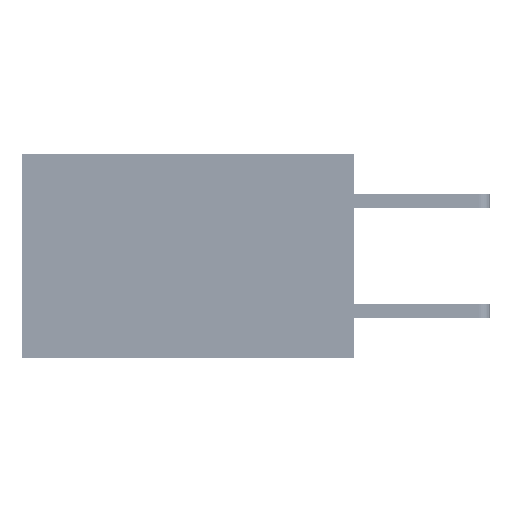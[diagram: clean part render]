
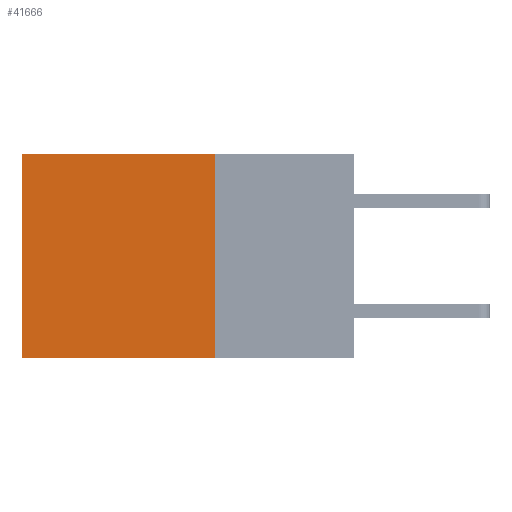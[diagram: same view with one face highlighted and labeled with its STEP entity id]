
A CAD part, left-side view. The second image highlights one B-rep face of the part: STEP entity #41666.
In plain terms, the highlighted planar face has unit normal (-1, 0, 0).
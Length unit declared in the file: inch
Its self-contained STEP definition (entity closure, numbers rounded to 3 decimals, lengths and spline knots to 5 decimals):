
#1092 = ORIENTED_EDGE ( 'NONE', *, *, #19078, .F. ) ;
#1303 = ORIENTED_EDGE ( 'NONE', *, *, #3907, .T. ) ;
#3804 = CARTESIAN_POINT ( 'NONE',  ( 0.2875, 0.25, 0. ) ) ;
#3907 = EDGE_CURVE ( 'NONE', #41631, #23849, #25362, .T. ) ;
#5537 = ORIENTED_EDGE ( 'NONE', *, *, #44155, .F. ) ;
#9464 = VECTOR ( 'NONE', #15674, 39.37008 ) ;
#11269 = ORIENTED_EDGE ( 'NONE', *, *, #43368, .T. ) ;
#11797 = CARTESIAN_POINT ( 'NONE',  ( 0.2875, 0.25, 0. ) ) ;
#15065 = VECTOR ( 'NONE', #29999, 39.37008 ) ;
#15167 = DIRECTION ( 'NONE',  ( 1., 0., 0. ) ) ;
#15674 = DIRECTION ( 'NONE',  ( 0., 0., -1. ) ) ;
#16047 = DIRECTION ( 'NONE',  ( 0., 0., -1. ) ) ;
#19078 = EDGE_CURVE ( 'NONE', #22400, #23849, #23038, .T. ) ;
#20884 = LINE ( 'NONE', #3804, #37593 ) ;
#21262 = CARTESIAN_POINT ( 'NONE',  ( 0.2875, 0.25, 0. ) ) ;
#21767 = CARTESIAN_POINT ( 'NONE',  ( 0.2875, 0.6, 0. ) ) ;
#22400 = VERTEX_POINT ( 'NONE', #25055 ) ;
#22505 = EDGE_LOOP ( 'NONE', ( #1303, #1092, #5537, #11269 ) ) ;
#22582 = CARTESIAN_POINT ( 'NONE',  ( 0.2875, 0.25, 0. ) ) ;
#23038 = LINE ( 'NONE', #36746, #15065 ) ;
#23849 = VERTEX_POINT ( 'NONE', #28532 ) ;
#23973 = DIRECTION ( 'NONE',  ( 0., 1., 0. ) ) ;
#24033 = DIRECTION ( 'NONE',  ( 0., 0., -1. ) ) ;
#24737 = AXIS2_PLACEMENT_3D ( 'NONE', #11797, #15167, #16047 ) ;
#25055 = CARTESIAN_POINT ( 'NONE',  ( 0.2875, 0.25, -0.37 ) ) ;
#25362 = LINE ( 'NONE', #21767, #9464 ) ;
#25516 = FACE_OUTER_BOUND ( 'NONE', #22505, .T. ) ;
#28532 = CARTESIAN_POINT ( 'NONE',  ( 0.2875, 0.6, -0.37 ) ) ;
#29999 = DIRECTION ( 'NONE',  ( 0., 1., 0. ) ) ;
#34093 = LINE ( 'NONE', #21262, #43367 ) ;
#36746 = CARTESIAN_POINT ( 'NONE',  ( 0.2875, 0.25, -0.37 ) ) ;
#37593 = VECTOR ( 'NONE', #24033, 39.37008 ) ;
#39455 = PLANE ( 'NONE',  #24737 ) ;
#41631 = VERTEX_POINT ( 'NONE', #42809 ) ;
#41666 = ADVANCED_FACE ( 'NONE', ( #25516 ), #39455, .F. ) ;
#41688 = VERTEX_POINT ( 'NONE', #22582 ) ;
#42809 = CARTESIAN_POINT ( 'NONE',  ( 0.2875, 0.6, 0. ) ) ;
#43367 = VECTOR ( 'NONE', #23973, 39.37008 ) ;
#43368 = EDGE_CURVE ( 'NONE', #41688, #41631, #34093, .T. ) ;
#44155 = EDGE_CURVE ( 'NONE', #41688, #22400, #20884, .T. ) ;
